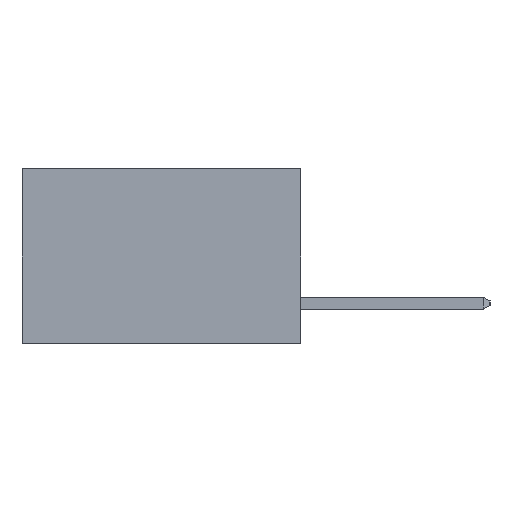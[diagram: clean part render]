
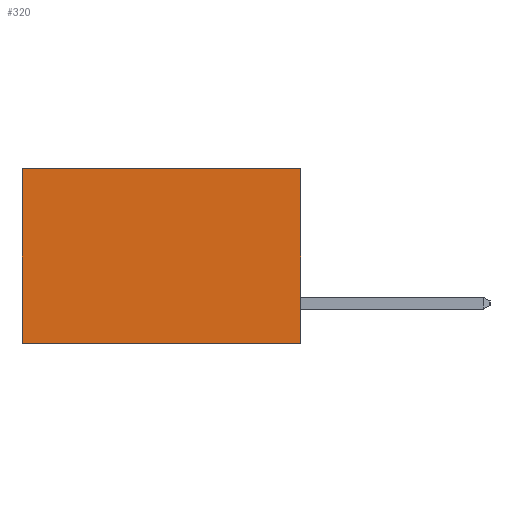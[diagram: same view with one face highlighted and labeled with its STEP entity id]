
A CAD part, left-side view. The second image highlights one B-rep face of the part: STEP entity #320.
In plain terms, the highlighted planar face has unit normal (-1, 0, 0).
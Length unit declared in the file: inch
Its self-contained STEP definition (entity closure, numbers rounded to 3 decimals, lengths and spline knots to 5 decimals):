
#320 = ADVANCED_FACE ( 'NONE', ( #9311 ), #14101, .F. ) ;
#649 = LINE ( 'NONE', #14097, #10386 ) ;
#842 = AXIS2_PLACEMENT_3D ( 'NONE', #4852, #4534, #5111 ) ;
#1154 = EDGE_CURVE ( 'NONE', #8397, #5651, #2880, .T. ) ;
#2569 = EDGE_CURVE ( 'NONE', #5651, #14653, #9185, .T. ) ;
#2880 = LINE ( 'NONE', #5891, #11950 ) ;
#3096 = CARTESIAN_POINT ( 'NONE',  ( 0.277, 0., -0.37 ) ) ;
#4534 = DIRECTION ( 'NONE',  ( 1., 0., 0. ) ) ;
#4852 = CARTESIAN_POINT ( 'NONE',  ( 0.277, 0., -0.37 ) ) ;
#4983 = ORIENTED_EDGE ( 'NONE', *, *, #5528, .F. ) ;
#5098 = CARTESIAN_POINT ( 'NONE',  ( 0.277, 0.59, -0.37 ) ) ;
#5111 = DIRECTION ( 'NONE',  ( 0., 0., -1. ) ) ;
#5528 = EDGE_CURVE ( 'NONE', #14003, #14653, #649, .T. ) ;
#5584 = EDGE_CURVE ( 'NONE', #8397, #14003, #13826, .T. ) ;
#5651 = VERTEX_POINT ( 'NONE', #12798 ) ;
#5891 = CARTESIAN_POINT ( 'NONE',  ( 0.277, 0., 0. ) ) ;
#7970 = EDGE_LOOP ( 'NONE', ( #9440, #4983, #10224, #10712 ) ) ;
#8397 = VERTEX_POINT ( 'NONE', #14048 ) ;
#9185 = LINE ( 'NONE', #12650, #14836 ) ;
#9311 = FACE_OUTER_BOUND ( 'NONE', #7970, .T. ) ;
#9440 = ORIENTED_EDGE ( 'NONE', *, *, #2569, .T. ) ;
#10224 = ORIENTED_EDGE ( 'NONE', *, *, #5584, .F. ) ;
#10386 = VECTOR ( 'NONE', #13963, 39.37008 ) ;
#10712 = ORIENTED_EDGE ( 'NONE', *, *, #1154, .T. ) ;
#11950 = VECTOR ( 'NONE', #14469, 39.37008 ) ;
#12650 = CARTESIAN_POINT ( 'NONE',  ( 0.277, 0.59, -0.37 ) ) ;
#12798 = CARTESIAN_POINT ( 'NONE',  ( 0.277, 0.59, 0. ) ) ;
#13462 = DIRECTION ( 'NONE',  ( 0., 0., -1. ) ) ;
#13473 = DIRECTION ( 'NONE',  ( 0., 0., -1. ) ) ;
#13477 = VECTOR ( 'NONE', #13473, 39.37008 ) ;
#13581 = CARTESIAN_POINT ( 'NONE',  ( 0.277, 0., -0.37 ) ) ;
#13826 = LINE ( 'NONE', #13581, #13477 ) ;
#13963 = DIRECTION ( 'NONE',  ( 0., 1., 0. ) ) ;
#14003 = VERTEX_POINT ( 'NONE', #3096 ) ;
#14048 = CARTESIAN_POINT ( 'NONE',  ( 0.277, 0., 0. ) ) ;
#14097 = CARTESIAN_POINT ( 'NONE',  ( 0.277, 0., -0.37 ) ) ;
#14101 = PLANE ( 'NONE',  #842 ) ;
#14469 = DIRECTION ( 'NONE',  ( 0., 1., 0. ) ) ;
#14653 = VERTEX_POINT ( 'NONE', #5098 ) ;
#14836 = VECTOR ( 'NONE', #13462, 39.37008 ) ;
